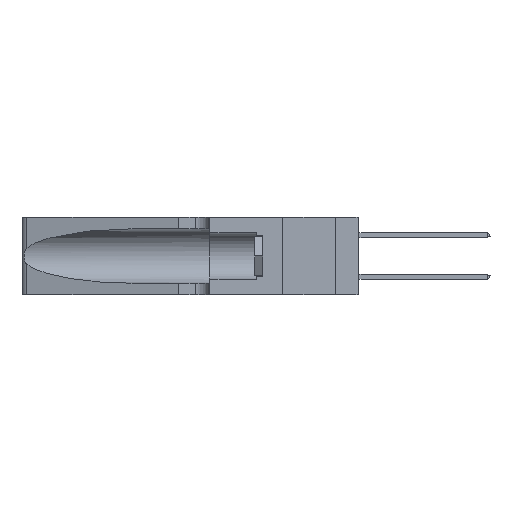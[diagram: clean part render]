
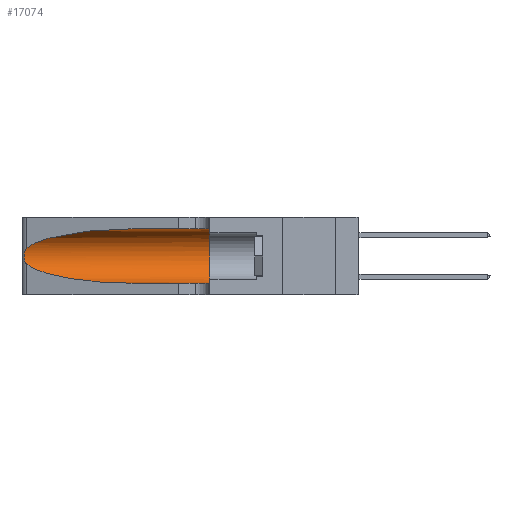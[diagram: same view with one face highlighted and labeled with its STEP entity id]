
A CAD part, left-side view. The second image highlights one B-rep face of the part: STEP entity #17074.
In plain terms, the highlighted cylindrical face has radius 3.308 mm (diameter 6.617 mm), a partial arc.
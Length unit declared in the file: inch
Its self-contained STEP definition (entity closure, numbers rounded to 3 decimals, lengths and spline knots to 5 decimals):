
#228 = VERTEX_POINT ( 'NONE', #13888 ) ;
#334 = CARTESIAN_POINT ( 'NONE',  ( 0.2373, 1.15595, 0.28018 ) ) ;
#571 = DIRECTION ( 'NONE',  ( 0., -1., 0. ) ) ;
#1862 = CARTESIAN_POINT ( 'NONE',  ( 0.25787, 1.23484, 0.2124 ) ) ;
#2857 = DIRECTION ( 'NONE',  ( 0., 1., 0. ) ) ;
#4401 = CARTESIAN_POINT ( 'NONE',  ( 0.2373, 1.15595, 0.08982 ) ) ;
#5194 = CARTESIAN_POINT ( 'NONE',  ( 0.26018, 1.23835, 0.19895 ) ) ;
#6519 = VERTEX_POINT ( 'NONE', #27876 ) ;
#6672 = VECTOR ( 'NONE', #29659, 39.37008 ) ;
#7264 = CARTESIAN_POINT ( 'NONE',  ( 0.1305, 1.61858, 0.185 ) ) ;
#7608 = ORIENTED_EDGE ( 'NONE', *, *, #20287, .T. ) ;
#7717 = CARTESIAN_POINT ( 'NONE',  ( 0.1305, 1.61858, 0.31525 ) ) ;
#7738 = CARTESIAN_POINT ( 'NONE',  ( 0.18966, 0.96281, 0.05475 ) ) ;
#8528 = CARTESIAN_POINT ( 'NONE',  ( 0.26075, 1.23896, 0.178 ) ) ;
#9456 = LINE ( 'NONE', #7717, #24580 ) ;
#9826 = AXIS2_PLACEMENT_3D ( 'NONE', #7264, #571, #29817 ) ;
#10213 = VERTEX_POINT ( 'NONE', #36646 ) ;
#11837 = CARTESIAN_POINT ( 'NONE',  ( 0.25856, 1.23593, 0.16098 ) ) ;
#12598 = CARTESIAN_POINT ( 'NONE',  ( 0.1305, 0.35, 0.05475 ) ) ;
#13568 = CARTESIAN_POINT ( 'NONE',  ( 0.1305, 1.61858, 0.05475 ) ) ;
#13888 = CARTESIAN_POINT ( 'NONE',  ( 0.1305, 0.72297, 0.31525 ) ) ;
#14041 = EDGE_CURVE ( 'NONE', #10213, #16112, #32270, .T. ) ;
#14351 =( BOUNDED_CURVE ( )  B_SPLINE_CURVE ( 3, ( #27029, #4401, #7738, #30267 ),
 .UNSPECIFIED., .F., .F. ) 
 B_SPLINE_CURVE_WITH_KNOTS ( ( 4, 4 ),
 ( 3.44316, 4.71239 ),
 .UNSPECIFIED. ) 
 CURVE ( )  GEOMETRIC_REPRESENTATION_ITEM ( )  RATIONAL_B_SPLINE_CURVE ( ( 1., 0.87, 0.87, 1. ) ) 
 REPRESENTATION_ITEM ( '' )  );
#14990 = CARTESIAN_POINT ( 'NONE',  ( 0.25487, 1.22718, 0.22369 ) ) ;
#15130 = CARTESIAN_POINT ( 'NONE',  ( 0.25639, 1.23186, 0.15144 ) ) ;
#15369 = LINE ( 'NONE', #13568, #6672 ) ;
#16112 = VERTEX_POINT ( 'NONE', #34560 ) ;
#16771 = CARTESIAN_POINT ( 'NONE',  ( 0.1305, 0.72297, 0.31525 ) ) ;
#17074 = ADVANCED_FACE ( 'NONE', ( #34976 ), #18082, .F. ) ;
#18082 = CYLINDRICAL_SURFACE ( 'NONE', #9826, 0.13025 ) ;
#18377 = CARTESIAN_POINT ( 'NONE',  ( 0.25487, 1.22718, 0.14631 ) ) ;
#19350 = ORIENTED_EDGE ( 'NONE', *, *, #30923, .F. ) ;
#19976 = CARTESIAN_POINT ( 'NONE',  ( 0.18966, 0.96281, 0.31525 ) ) ;
#20060 = VERTEX_POINT ( 'NONE', #12598 ) ;
#20287 = EDGE_CURVE ( 'NONE', #6519, #20060, #15369, .T. ) ;
#20750 = EDGE_CURVE ( 'NONE', #21167, #20060, #21838, .T. ) ;
#21167 = VERTEX_POINT ( 'NONE', #37878 ) ;
#21448 = CARTESIAN_POINT ( 'NONE',  ( 0.25639, 1.23184, 0.21858 ) ) ;
#21814 = ORIENTED_EDGE ( 'NONE', *, *, #14041, .T. ) ;
#21825 =( BOUNDED_CURVE ( )  B_SPLINE_CURVE ( 3, ( #16771, #19976, #334, #23189 ),
 .UNSPECIFIED., .F., .F. ) 
 B_SPLINE_CURVE_WITH_KNOTS ( ( 4, 4 ),
 ( 1.5708, 2.84003 ),
 .UNSPECIFIED. ) 
 CURVE ( )  GEOMETRIC_REPRESENTATION_ITEM ( )  RATIONAL_B_SPLINE_CURVE ( ( 1., 0.87, 0.87, 1. ) ) 
 REPRESENTATION_ITEM ( '' )  );
#21838 = CIRCLE ( 'NONE', #40438, 0.13025 ) ;
#22385 = CARTESIAN_POINT ( 'NONE',  ( 0.1305, 0.35, 0.185 ) ) ;
#23189 = CARTESIAN_POINT ( 'NONE',  ( 0.25487, 1.22718, 0.22369 ) ) ;
#24310 = EDGE_LOOP ( 'NONE', ( #37682, #21814, #32259, #7608, #26770, #19350 ) ) ;
#24580 = VECTOR ( 'NONE', #36588, 39.37008 ) ;
#24631 = CARTESIAN_POINT ( 'NONE',  ( 0.25854, 1.2359, 0.20912 ) ) ;
#25557 = DIRECTION ( 'NONE',  ( 0., 0., 1. ) ) ;
#26770 = ORIENTED_EDGE ( 'NONE', *, *, #20750, .F. ) ;
#27029 = CARTESIAN_POINT ( 'NONE',  ( 0.25487, 1.22718, 0.14631 ) ) ;
#27804 = CARTESIAN_POINT ( 'NONE',  ( 0.26075, 1.23896, 0.19203 ) ) ;
#27876 = CARTESIAN_POINT ( 'NONE',  ( 0.1305, 0.72297, 0.05475 ) ) ;
#29659 = DIRECTION ( 'NONE',  ( 0., -1., 0. ) ) ;
#29817 = DIRECTION ( 'NONE',  ( 0., 0., -1. ) ) ;
#30267 = CARTESIAN_POINT ( 'NONE',  ( 0.1305, 0.72297, 0.05475 ) ) ;
#30923 = EDGE_CURVE ( 'NONE', #228, #21167, #9456, .T. ) ;
#31019 = CARTESIAN_POINT ( 'NONE',  ( 0.26017, 1.23833, 0.17102 ) ) ;
#32259 = ORIENTED_EDGE ( 'NONE', *, *, #34741, .T. ) ;
#32270 = B_SPLINE_CURVE_WITH_KNOTS ( 'NONE', 3,
 ( #14990, #40456, #21448, #1862, #24631, #5194, #27804, #8528, #31019, #11837, #34184, #15130, #37367, #18377 ),
 .UNSPECIFIED., .F., .F.,
 ( 4, 2, 2, 2, 2, 2, 4 ),
 ( 0., 0.00027, 0.00053, 0.00107, 0.0016, 0.00187, 0.00214 ),
 .UNSPECIFIED. ) ;
#32683 = EDGE_CURVE ( 'NONE', #228, #10213, #21825, .T. ) ;
#34184 = CARTESIAN_POINT ( 'NONE',  ( 0.25789, 1.23486, 0.15765 ) ) ;
#34560 = CARTESIAN_POINT ( 'NONE',  ( 0.25487, 1.22718, 0.14631 ) ) ;
#34741 = EDGE_CURVE ( 'NONE', #16112, #6519, #14351, .T. ) ;
#34976 = FACE_OUTER_BOUND ( 'NONE', #24310, .T. ) ;
#36588 = DIRECTION ( 'NONE',  ( 0., -1., 0. ) ) ;
#36646 = CARTESIAN_POINT ( 'NONE',  ( 0.25487, 1.22718, 0.22369 ) ) ;
#37367 = CARTESIAN_POINT ( 'NONE',  ( 0.25555, 1.22993, 0.14849 ) ) ;
#37682 = ORIENTED_EDGE ( 'NONE', *, *, #32683, .T. ) ;
#37878 = CARTESIAN_POINT ( 'NONE',  ( 0.1305, 0.35, 0.31525 ) ) ;
#40438 = AXIS2_PLACEMENT_3D ( 'NONE', #22385, #2857, #25557 ) ;
#40456 = CARTESIAN_POINT ( 'NONE',  ( 0.25555, 1.22994, 0.2215 ) ) ;
